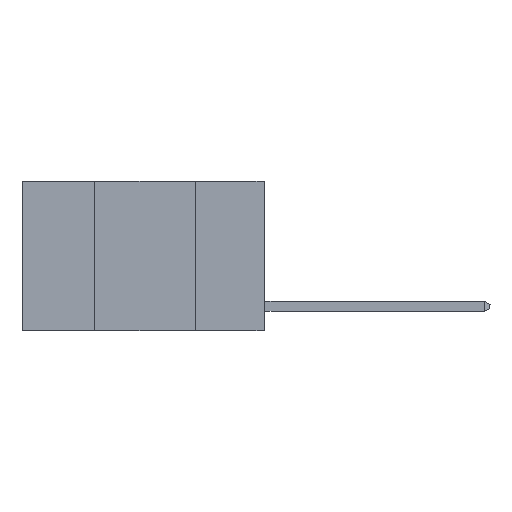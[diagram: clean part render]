
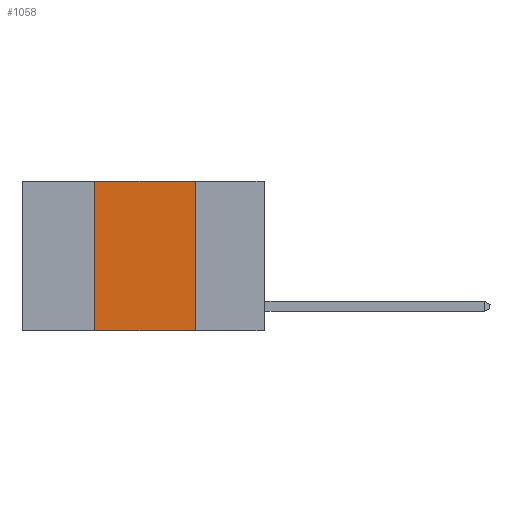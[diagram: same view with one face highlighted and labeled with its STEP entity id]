
A CAD part, left-side view. The second image highlights one B-rep face of the part: STEP entity #1058.
In plain terms, the highlighted planar face has unit normal (-1, 0, 0).
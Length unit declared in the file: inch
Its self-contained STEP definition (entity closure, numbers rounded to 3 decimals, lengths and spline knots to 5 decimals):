
#652 = DIRECTION ( 'NONE',  ( 0., -1., 0. ) ) ;
#756 = DIRECTION ( 'NONE',  ( 0., 0., 1. ) ) ;
#863 = EDGE_LOOP ( 'NONE', ( #16264, #24768, #981, #15477 ) ) ;
#981 = ORIENTED_EDGE ( 'NONE', *, *, #12703, .F. ) ;
#1058 = ADVANCED_FACE ( 'NONE', ( #7599 ), #18263, .F. ) ;
#1072 = VECTOR ( 'NONE', #2076, 39.37008 ) ;
#1342 = VERTEX_POINT ( 'NONE', #27105 ) ;
#2076 = DIRECTION ( 'NONE',  ( 0., 0., -1. ) ) ;
#2271 = VERTEX_POINT ( 'NONE', #3960 ) ;
#2444 = VERTEX_POINT ( 'NONE', #3697 ) ;
#3697 = CARTESIAN_POINT ( 'NONE',  ( 0., 0.42, -0.37 ) ) ;
#3960 = CARTESIAN_POINT ( 'NONE',  ( 0., 0.17, 0. ) ) ;
#4978 = LINE ( 'NONE', #11487, #20322 ) ;
#6057 = CARTESIAN_POINT ( 'NONE',  ( 0., 0.6, 0. ) ) ;
#7599 = FACE_OUTER_BOUND ( 'NONE', #863, .T. ) ;
#11487 = CARTESIAN_POINT ( 'NONE',  ( 0., 0.6, -0.37 ) ) ;
#12703 = EDGE_CURVE ( 'NONE', #2444, #24718, #21293, .T. ) ;
#13692 = CARTESIAN_POINT ( 'NONE',  ( 0., 0.42, 0. ) ) ;
#15122 = CARTESIAN_POINT ( 'NONE',  ( 0., 0.17, 0. ) ) ;
#15477 = ORIENTED_EDGE ( 'NONE', *, *, #20078, .T. ) ;
#16264 = ORIENTED_EDGE ( 'NONE', *, *, #16759, .F. ) ;
#16669 = DIRECTION ( 'NONE',  ( 1., 0., 0. ) ) ;
#16759 = EDGE_CURVE ( 'NONE', #2271, #1342, #17761, .T. ) ;
#17424 = CARTESIAN_POINT ( 'NONE',  ( 0., 0.6, 0. ) ) ;
#17761 = LINE ( 'NONE', #15122, #1072 ) ;
#18263 = PLANE ( 'NONE',  #24831 ) ;
#18928 = VECTOR ( 'NONE', #27745, 39.37008 ) ;
#19529 = CARTESIAN_POINT ( 'NONE',  ( 0., 0.42, 0. ) ) ;
#20078 = EDGE_CURVE ( 'NONE', #2444, #1342, #4978, .T. ) ;
#20322 = VECTOR ( 'NONE', #652, 39.37008 ) ;
#21293 = LINE ( 'NONE', #13692, #26366 ) ;
#23240 = DIRECTION ( 'NONE',  ( 0., 0., -1. ) ) ;
#23364 = EDGE_CURVE ( 'NONE', #24718, #2271, #25359, .T. ) ;
#24718 = VERTEX_POINT ( 'NONE', #19529 ) ;
#24768 = ORIENTED_EDGE ( 'NONE', *, *, #23364, .F. ) ;
#24831 = AXIS2_PLACEMENT_3D ( 'NONE', #17424, #16669, #23240 ) ;
#25359 = LINE ( 'NONE', #6057, #18928 ) ;
#26366 = VECTOR ( 'NONE', #756, 39.37008 ) ;
#27105 = CARTESIAN_POINT ( 'NONE',  ( 0., 0.17, -0.37 ) ) ;
#27745 = DIRECTION ( 'NONE',  ( 0., -1., 0. ) ) ;
